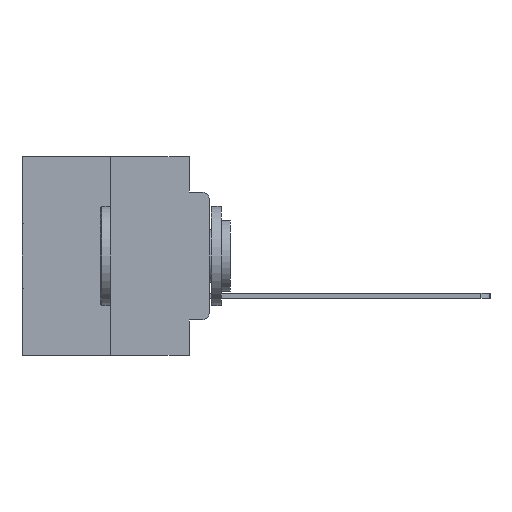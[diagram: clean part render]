
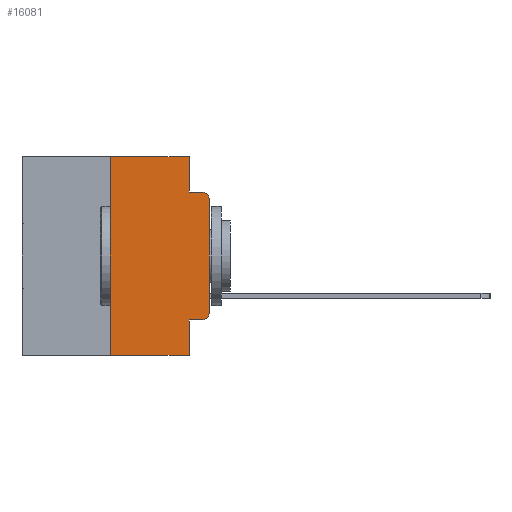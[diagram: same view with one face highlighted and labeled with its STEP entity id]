
A CAD part, left-side view. The second image highlights one B-rep face of the part: STEP entity #16081.
In plain terms, the highlighted planar face has unit normal (-1, 0, 0).
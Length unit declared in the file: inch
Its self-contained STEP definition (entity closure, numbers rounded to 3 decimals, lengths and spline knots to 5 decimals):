
#43 = ORIENTED_EDGE ( 'NONE', *, *, #6390, .T. ) ;
#203 = CARTESIAN_POINT ( 'NONE',  ( 0., 0.051, 0. ) ) ;
#218 = DIRECTION ( 'NONE',  ( 0., 0., -1. ) ) ;
#229 = VERTEX_POINT ( 'NONE', #28643 ) ;
#461 = ORIENTED_EDGE ( 'NONE', *, *, #26813, .F. ) ;
#634 = CARTESIAN_POINT ( 'NONE',  ( 0., 0., -0.1085 ) ) ;
#1668 = CARTESIAN_POINT ( 'NONE',  ( 0., 0.25, -0.5 ) ) ;
#2333 = ORIENTED_EDGE ( 'NONE', *, *, #23785, .F. ) ;
#2463 = AXIS2_PLACEMENT_3D ( 'NONE', #10279, #5783, #21780 ) ;
#2664 = LINE ( 'NONE', #4612, #20929 ) ;
#2961 = VECTOR ( 'NONE', #27330, 39.37008 ) ;
#3342 = VERTEX_POINT ( 'NONE', #21984 ) ;
#3386 = DIRECTION ( 'NONE',  ( -1., 0., 0. ) ) ;
#4159 = VECTOR ( 'NONE', #22556, 39.37008 ) ;
#4405 = AXIS2_PLACEMENT_3D ( 'NONE', #17132, #3386, #19423 ) ;
#4612 = CARTESIAN_POINT ( 'NONE',  ( 0., 0.473, 0. ) ) ;
#4852 = EDGE_CURVE ( 'NONE', #9789, #9065, #11672, .T. ) ;
#5783 = DIRECTION ( 'NONE',  ( 1., 0., 0. ) ) ;
#5991 = CARTESIAN_POINT ( 'NONE',  ( 0., 0.051, -0.0885 ) ) ;
#6390 = EDGE_CURVE ( 'NONE', #13788, #9789, #15179, .T. ) ;
#6580 = CARTESIAN_POINT ( 'NONE',  ( 0., 0.051, -0.4115 ) ) ;
#7097 = DIRECTION ( 'NONE',  ( 0., 0., -1. ) ) ;
#7595 = VERTEX_POINT ( 'NONE', #27163 ) ;
#7981 = PLANE ( 'NONE',  #2463 ) ;
#8374 = AXIS2_PLACEMENT_3D ( 'NONE', #27521, #13967, #218 ) ;
#8663 = VERTEX_POINT ( 'NONE', #17958 ) ;
#9065 = VERTEX_POINT ( 'NONE', #19427 ) ;
#9136 = LINE ( 'NONE', #203, #27275 ) ;
#9347 = VECTOR ( 'NONE', #23572, 39.37008 ) ;
#9789 = VERTEX_POINT ( 'NONE', #634 ) ;
#10229 = LINE ( 'NONE', #6580, #4159 ) ;
#10238 = EDGE_CURVE ( 'NONE', #8663, #229, #2664, .T. ) ;
#10279 = CARTESIAN_POINT ( 'NONE',  ( 0., 0.473, 0. ) ) ;
#10641 = CARTESIAN_POINT ( 'NONE',  ( 0., 0.051, -0.4115 ) ) ;
#10692 = CIRCLE ( 'NONE', #4405, 0.02 ) ;
#10797 = DIRECTION ( 'NONE',  ( 0., 0., 1. ) ) ;
#10945 = LINE ( 'NONE', #19933, #22375 ) ;
#11672 = CIRCLE ( 'NONE', #8374, 0.02 ) ;
#11708 = EDGE_LOOP ( 'NONE', ( #43, #25045, #11906, #461, #14102, #29314, #13441, #2333, #19642, #14236 ) ) ;
#11906 = ORIENTED_EDGE ( 'NONE', *, *, #28279, .F. ) ;
#13441 = ORIENTED_EDGE ( 'NONE', *, *, #24170, .T. ) ;
#13788 = VERTEX_POINT ( 'NONE', #26212 ) ;
#13967 = DIRECTION ( 'NONE',  ( -1., 0., 0. ) ) ;
#14102 = ORIENTED_EDGE ( 'NONE', *, *, #10238, .F. ) ;
#14236 = ORIENTED_EDGE ( 'NONE', *, *, #19273, .T. ) ;
#15179 = LINE ( 'NONE', #25054, #2961 ) ;
#15200 = VECTOR ( 'NONE', #10797, 39.37008 ) ;
#16058 = DIRECTION ( 'NONE',  ( 0., -1., 0. ) ) ;
#16081 = ADVANCED_FACE ( 'NONE', ( #22286 ), #7981, .F. ) ;
#16198 = VERTEX_POINT ( 'NONE', #1668 ) ;
#16793 = VERTEX_POINT ( 'NONE', #10641 ) ;
#17132 = CARTESIAN_POINT ( 'NONE',  ( 0., 0.02, -0.3915 ) ) ;
#17351 = CARTESIAN_POINT ( 'NONE',  ( 0., 0.051, -0.0885 ) ) ;
#17958 = CARTESIAN_POINT ( 'NONE',  ( 0., 0.25, 0. ) ) ;
#18066 = LINE ( 'NONE', #5991, #29277 ) ;
#19057 = CARTESIAN_POINT ( 'NONE',  ( 0., 0.051, 0. ) ) ;
#19273 = EDGE_CURVE ( 'NONE', #3342, #13788, #10692, .T. ) ;
#19423 = DIRECTION ( 'NONE',  ( 0., 0., -1. ) ) ;
#19427 = CARTESIAN_POINT ( 'NONE',  ( 0., 0.02, -0.0885 ) ) ;
#19642 = ORIENTED_EDGE ( 'NONE', *, *, #20771, .T. ) ;
#19729 = DIRECTION ( 'NONE',  ( 0., -1., 0. ) ) ;
#19933 = CARTESIAN_POINT ( 'NONE',  ( 0., 0.473, -0.5 ) ) ;
#20771 = EDGE_CURVE ( 'NONE', #16793, #3342, #10229, .T. ) ;
#20929 = VECTOR ( 'NONE', #16058, 39.37008 ) ;
#21780 = DIRECTION ( 'NONE',  ( 0., 0., -1. ) ) ;
#21984 = CARTESIAN_POINT ( 'NONE',  ( 0., 0.02, -0.4115 ) ) ;
#22182 = CARTESIAN_POINT ( 'NONE',  ( 0., 0.25, 0. ) ) ;
#22286 = FACE_OUTER_BOUND ( 'NONE', #11708, .T. ) ;
#22375 = VECTOR ( 'NONE', #28931, 39.37008 ) ;
#22556 = DIRECTION ( 'NONE',  ( 0., -1., 0. ) ) ;
#23572 = DIRECTION ( 'NONE',  ( 0., 0., -1. ) ) ;
#23785 = EDGE_CURVE ( 'NONE', #16793, #7595, #9136, .T. ) ;
#24067 = VERTEX_POINT ( 'NONE', #17351 ) ;
#24170 = EDGE_CURVE ( 'NONE', #16198, #7595, #10945, .T. ) ;
#25045 = ORIENTED_EDGE ( 'NONE', *, *, #4852, .T. ) ;
#25054 = CARTESIAN_POINT ( 'NONE',  ( 0., 0., 0. ) ) ;
#25282 = EDGE_CURVE ( 'NONE', #16198, #8663, #28601, .T. ) ;
#26212 = CARTESIAN_POINT ( 'NONE',  ( 0., 0., -0.3915 ) ) ;
#26813 = EDGE_CURVE ( 'NONE', #229, #24067, #27480, .T. ) ;
#27163 = CARTESIAN_POINT ( 'NONE',  ( 0., 0.051, -0.5 ) ) ;
#27275 = VECTOR ( 'NONE', #7097, 39.37008 ) ;
#27330 = DIRECTION ( 'NONE',  ( 0., 0., 1. ) ) ;
#27480 = LINE ( 'NONE', #19057, #9347 ) ;
#27521 = CARTESIAN_POINT ( 'NONE',  ( 0., 0.02, -0.1085 ) ) ;
#28279 = EDGE_CURVE ( 'NONE', #24067, #9065, #18066, .T. ) ;
#28601 = LINE ( 'NONE', #22182, #15200 ) ;
#28643 = CARTESIAN_POINT ( 'NONE',  ( 0., 0.051, 0. ) ) ;
#28931 = DIRECTION ( 'NONE',  ( 0., -1., 0. ) ) ;
#29277 = VECTOR ( 'NONE', #19729, 39.37008 ) ;
#29314 = ORIENTED_EDGE ( 'NONE', *, *, #25282, .F. ) ;
